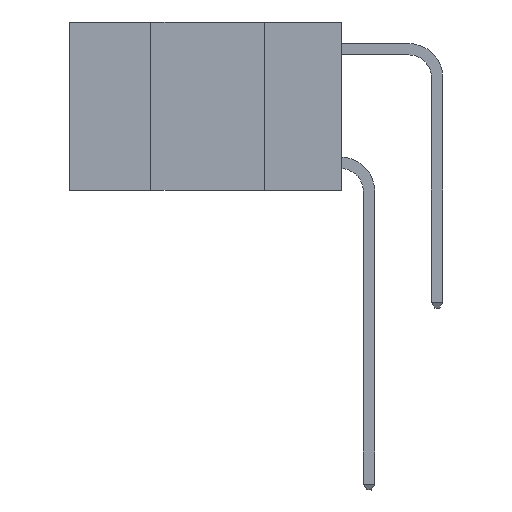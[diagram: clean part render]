
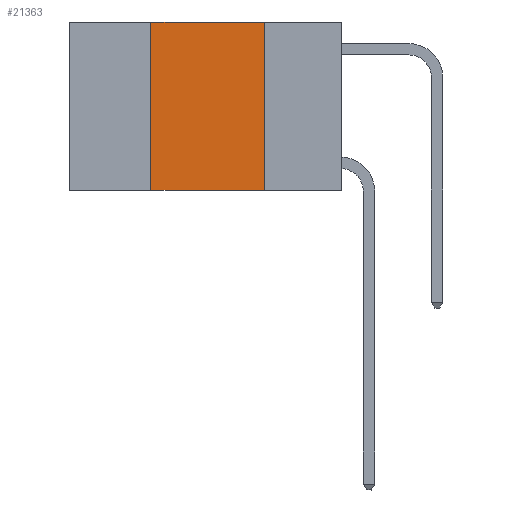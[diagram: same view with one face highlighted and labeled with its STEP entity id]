
A CAD part, left-side view. The second image highlights one B-rep face of the part: STEP entity #21363.
In plain terms, the highlighted planar face has unit normal (-1, 0, 0).
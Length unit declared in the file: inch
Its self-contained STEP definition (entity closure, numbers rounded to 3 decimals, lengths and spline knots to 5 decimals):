
#312 = VECTOR ( 'NONE', #17404, 39.37008 ) ;
#382 = VECTOR ( 'NONE', #20004, 39.37008 ) ;
#1178 = DIRECTION ( 'NONE',  ( 0., 0., -1. ) ) ;
#2819 = CARTESIAN_POINT ( 'NONE',  ( 0., 0.42, 0. ) ) ;
#3133 = VERTEX_POINT ( 'NONE', #11666 ) ;
#3855 = CARTESIAN_POINT ( 'NONE',  ( 0., 0.42, -0.37 ) ) ;
#3911 = ORIENTED_EDGE ( 'NONE', *, *, #10462, .T. ) ;
#3927 = VECTOR ( 'NONE', #10794, 39.37008 ) ;
#4380 = CARTESIAN_POINT ( 'NONE',  ( 0., 0.17, 0. ) ) ;
#4728 = ORIENTED_EDGE ( 'NONE', *, *, #4984, .F. ) ;
#4984 = EDGE_CURVE ( 'NONE', #9983, #22187, #5479, .T. ) ;
#5105 = EDGE_CURVE ( 'NONE', #22187, #12110, #17760, .T. ) ;
#5209 = DIRECTION ( 'NONE',  ( 0., -1., 0. ) ) ;
#5395 = ORIENTED_EDGE ( 'NONE', *, *, #14880, .F. ) ;
#5479 = LINE ( 'NONE', #2819, #382 ) ;
#5826 = AXIS2_PLACEMENT_3D ( 'NONE', #10824, #12734, #1178 ) ;
#9805 = CARTESIAN_POINT ( 'NONE',  ( 0., 0.17, 0. ) ) ;
#9983 = VERTEX_POINT ( 'NONE', #3855 ) ;
#10462 = EDGE_CURVE ( 'NONE', #9983, #3133, #14634, .T. ) ;
#10615 = CARTESIAN_POINT ( 'NONE',  ( 0., 0.6, -0.37 ) ) ;
#10794 = DIRECTION ( 'NONE',  ( 0., -1., 0. ) ) ;
#10824 = CARTESIAN_POINT ( 'NONE',  ( 0., 0.6, 0. ) ) ;
#11666 = CARTESIAN_POINT ( 'NONE',  ( 0., 0.17, -0.37 ) ) ;
#12110 = VERTEX_POINT ( 'NONE', #4380 ) ;
#12734 = DIRECTION ( 'NONE',  ( 1., 0., 0. ) ) ;
#14634 = LINE ( 'NONE', #10615, #21615 ) ;
#14880 = EDGE_CURVE ( 'NONE', #12110, #3133, #24327, .T. ) ;
#16957 = FACE_OUTER_BOUND ( 'NONE', #17196, .T. ) ;
#17196 = EDGE_LOOP ( 'NONE', ( #5395, #17933, #4728, #3911 ) ) ;
#17404 = DIRECTION ( 'NONE',  ( 0., 0., -1. ) ) ;
#17760 = LINE ( 'NONE', #22355, #3927 ) ;
#17933 = ORIENTED_EDGE ( 'NONE', *, *, #5105, .F. ) ;
#20004 = DIRECTION ( 'NONE',  ( 0., 0., 1. ) ) ;
#21363 = ADVANCED_FACE ( 'NONE', ( #16957 ), #24063, .F. ) ;
#21615 = VECTOR ( 'NONE', #5209, 39.37008 ) ;
#22187 = VERTEX_POINT ( 'NONE', #23017 ) ;
#22355 = CARTESIAN_POINT ( 'NONE',  ( 0., 0.6, 0. ) ) ;
#23017 = CARTESIAN_POINT ( 'NONE',  ( 0., 0.42, 0. ) ) ;
#24063 = PLANE ( 'NONE',  #5826 ) ;
#24327 = LINE ( 'NONE', #9805, #312 ) ;
